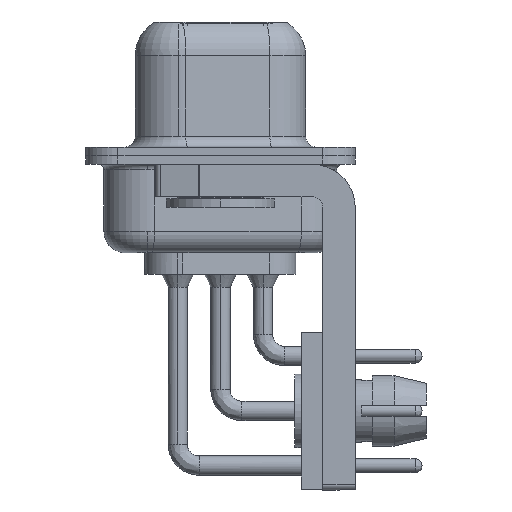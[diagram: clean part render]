
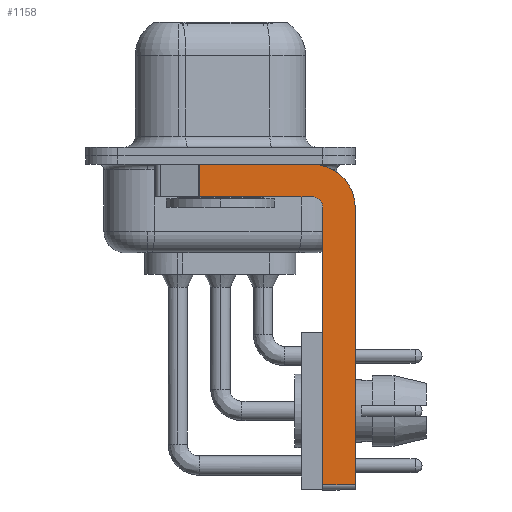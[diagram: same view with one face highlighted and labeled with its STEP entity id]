
A CAD part, left-side view. The second image highlights one B-rep face of the part: STEP entity #1158.
In plain terms, the highlighted planar face has unit normal (-1, 0, 0).
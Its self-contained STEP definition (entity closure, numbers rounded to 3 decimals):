
#53 = VERTEX_POINT ( 'NONE', #8704 ) ;
#267 = VERTEX_POINT ( 'NONE', #16775 ) ;
#275 = CARTESIAN_POINT ( 'NONE',  ( -2.9, -4.25, -15.25 ) ) ;
#777 = CIRCLE ( 'NONE', #16646, 2. ) ;
#1158 = ADVANCED_FACE ( 'NONE', ( #9061 ), #11013, .F. ) ;
#1167 = EDGE_CURVE ( 'NONE', #9131, #53, #14269, .T. ) ;
#1483 = CARTESIAN_POINT ( 'NONE',  ( -2.9, -4.75, -15.5 ) ) ;
#1547 = EDGE_CURVE ( 'NONE', #6457, #267, #19110, .T. ) ;
#1984 = LINE ( 'NONE', #275, #7822 ) ;
#3311 = LINE ( 'NONE', #1483, #15082 ) ;
#4465 = DIRECTION ( 'NONE',  ( -1., 0., 0. ) ) ;
#4584 = CARTESIAN_POINT ( 'NONE',  ( -2.9, -6.25, -2.4 ) ) ;
#4636 = EDGE_CURVE ( 'NONE', #23199, #7116, #24791, .T. ) ;
#5746 = ORIENTED_EDGE ( 'NONE', *, *, #6870, .F. ) ;
#5751 = EDGE_CURVE ( 'NONE', #19598, #7116, #1984, .T. ) ;
#6457 = VERTEX_POINT ( 'NONE', #22231 ) ;
#6596 = VECTOR ( 'NONE', #23614, 1000. ) ;
#6870 = EDGE_CURVE ( 'NONE', #19598, #27752, #3311, .T. ) ;
#6975 = AXIS2_PLACEMENT_3D ( 'NONE', #10906, #15243, #11413 ) ;
#7116 = VERTEX_POINT ( 'NONE', #15654 ) ;
#7126 = ORIENTED_EDGE ( 'NONE', *, *, #9089, .F. ) ;
#7822 = VECTOR ( 'NONE', #13491, 1000. ) ;
#8704 = CARTESIAN_POINT ( 'NONE',  ( -2.9, -4.25, -0.4 ) ) ;
#9061 = FACE_OUTER_BOUND ( 'NONE', #18436, .T. ) ;
#9089 = EDGE_CURVE ( 'NONE', #27752, #6457, #26948, .T. ) ;
#9131 = VERTEX_POINT ( 'NONE', #17957 ) ;
#9520 = CARTESIAN_POINT ( 'NONE',  ( -2.9, -4.75, -15.25 ) ) ;
#9680 = AXIS2_PLACEMENT_3D ( 'NONE', #17767, #4465, #19951 ) ;
#9685 = CARTESIAN_POINT ( 'NONE',  ( -2.9, -6.25, -2.4 ) ) ;
#10781 = DIRECTION ( 'NONE',  ( 1., 0., 0. ) ) ;
#10906 = CARTESIAN_POINT ( 'NONE',  ( -2.9, -4.25, -2.4 ) ) ;
#11013 = PLANE ( 'NONE',  #6975 ) ;
#11219 = CARTESIAN_POINT ( 'NONE',  ( -2.9, 3., -0.4 ) ) ;
#11374 = DIRECTION ( 'NONE',  ( 0., -1., 0. ) ) ;
#11413 = DIRECTION ( 'NONE',  ( 0., 0., -1. ) ) ;
#12717 = ORIENTED_EDGE ( 'NONE', *, *, #27920, .F. ) ;
#12905 = ORIENTED_EDGE ( 'NONE', *, *, #14129, .T. ) ;
#13491 = DIRECTION ( 'NONE',  ( 0., -1., 0. ) ) ;
#14129 = EDGE_CURVE ( 'NONE', #9131, #267, #26343, .T. ) ;
#14269 = LINE ( 'NONE', #11219, #19459 ) ;
#14378 = DIRECTION ( 'NONE',  ( 0., 0., -1. ) ) ;
#15082 = VECTOR ( 'NONE', #25739, 1000. ) ;
#15243 = DIRECTION ( 'NONE',  ( 1., 0., 0. ) ) ;
#15654 = CARTESIAN_POINT ( 'NONE',  ( -2.9, -6.25, -15.25 ) ) ;
#16191 = ORIENTED_EDGE ( 'NONE', *, *, #5751, .T. ) ;
#16646 = AXIS2_PLACEMENT_3D ( 'NONE', #23982, #10781, #26181 ) ;
#16775 = CARTESIAN_POINT ( 'NONE',  ( -2.9, 0.978, -1.9 ) ) ;
#17244 = ORIENTED_EDGE ( 'NONE', *, *, #1167, .F. ) ;
#17767 = CARTESIAN_POINT ( 'NONE',  ( -2.9, -4.25, -2.4 ) ) ;
#17957 = CARTESIAN_POINT ( 'NONE',  ( -2.9, 0.978, -0.4 ) ) ;
#18314 = VECTOR ( 'NONE', #20709, 1000. ) ;
#18436 = EDGE_LOOP ( 'NONE', ( #17244, #12905, #22924, #7126, #5746, #16191, #22398, #12717 ) ) ;
#19110 = LINE ( 'NONE', #23342, #6596 ) ;
#19459 = VECTOR ( 'NONE', #11374, 1000. ) ;
#19598 = VERTEX_POINT ( 'NONE', #9520 ) ;
#19951 = DIRECTION ( 'NONE',  ( 0., 0., 1. ) ) ;
#20544 = VECTOR ( 'NONE', #14378, 1000. ) ;
#20709 = DIRECTION ( 'NONE',  ( 0., 0., -1. ) ) ;
#22231 = CARTESIAN_POINT ( 'NONE',  ( -2.9, -4.25, -1.9 ) ) ;
#22398 = ORIENTED_EDGE ( 'NONE', *, *, #4636, .F. ) ;
#22924 = ORIENTED_EDGE ( 'NONE', *, *, #1547, .F. ) ;
#23199 = VERTEX_POINT ( 'NONE', #4584 ) ;
#23342 = CARTESIAN_POINT ( 'NONE',  ( -2.9, -4.25, -1.9 ) ) ;
#23435 = CARTESIAN_POINT ( 'NONE',  ( -2.9, -4.75, -2.4 ) ) ;
#23614 = DIRECTION ( 'NONE',  ( 0., 1., 0. ) ) ;
#23982 = CARTESIAN_POINT ( 'NONE',  ( -2.9, -4.25, -2.4 ) ) ;
#24791 = LINE ( 'NONE', #9685, #18314 ) ;
#25335 = CARTESIAN_POINT ( 'NONE',  ( -2.9, 0.978, -1.9 ) ) ;
#25739 = DIRECTION ( 'NONE',  ( 0., 0., 1. ) ) ;
#26181 = DIRECTION ( 'NONE',  ( 0., 0., -1. ) ) ;
#26343 = LINE ( 'NONE', #25335, #20544 ) ;
#26948 = CIRCLE ( 'NONE', #9680, 0.5 ) ;
#27752 = VERTEX_POINT ( 'NONE', #23435 ) ;
#27920 = EDGE_CURVE ( 'NONE', #53, #23199, #777, .T. ) ;
